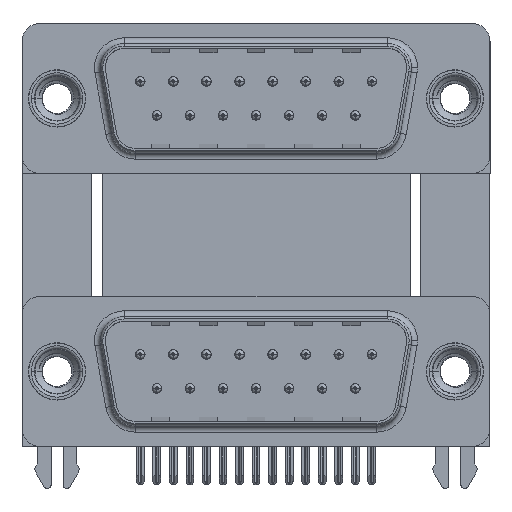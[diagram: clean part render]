
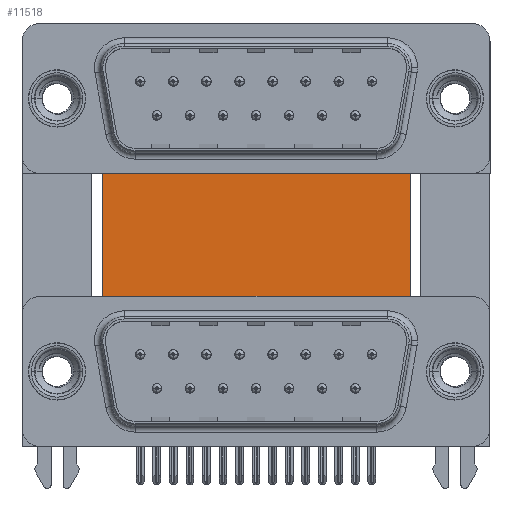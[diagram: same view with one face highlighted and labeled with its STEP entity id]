
A CAD part, top view. The second image highlights one B-rep face of the part: STEP entity #11518.
In plain terms, the highlighted planar face has unit normal (0, 0, 1).
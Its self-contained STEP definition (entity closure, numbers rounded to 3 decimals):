
#62 = VERTEX_POINT ( 'NONE', #31381 ) ;
#1305 = LINE ( 'NONE', #28938, #19242 ) ;
#3365 = CARTESIAN_POINT ( 'NONE',  ( 3.79, 16.585, -12. ) ) ;
#4506 = LINE ( 'NONE', #14262, #23867 ) ;
#5731 = PLANE ( 'NONE',  #9379 ) ;
#6232 = FACE_OUTER_BOUND ( 'NONE', #24358, .T. ) ;
#8092 = DIRECTION ( 'NONE',  ( 0., -1., 0. ) ) ;
#8930 = DIRECTION ( 'NONE',  ( 0., 0., -1. ) ) ;
#9379 = AXIS2_PLACEMENT_3D ( 'NONE', #19197, #8930, #10949 ) ;
#9506 = LINE ( 'NONE', #32763, #24781 ) ;
#10602 = LINE ( 'NONE', #3365, #31676 ) ;
#10753 = EDGE_CURVE ( 'NONE', #26632, #62, #4506, .T. ) ;
#10949 = DIRECTION ( 'NONE',  ( -1., 0., 0. ) ) ;
#11046 = ORIENTED_EDGE ( 'NONE', *, *, #25120, .F. ) ;
#11518 = ADVANCED_FACE ( 'NONE', ( #6232 ), #5731, .F. ) ;
#14262 = CARTESIAN_POINT ( 'NONE',  ( 3.79, -3.735, -12. ) ) ;
#14571 = DIRECTION ( 'NONE',  ( 0., -1., 0. ) ) ;
#14952 = ORIENTED_EDGE ( 'NONE', *, *, #10753, .T. ) ;
#16306 = EDGE_CURVE ( 'NONE', #31346, #26551, #1305, .T. ) ;
#16488 = CARTESIAN_POINT ( 'NONE',  ( 3.79, 16.585, -12. ) ) ;
#16693 = ORIENTED_EDGE ( 'NONE', *, *, #26308, .T. ) ;
#16793 = DIRECTION ( 'NONE',  ( 1., 0., 0. ) ) ;
#17887 = ORIENTED_EDGE ( 'NONE', *, *, #16306, .F. ) ;
#19197 = CARTESIAN_POINT ( 'NONE',  ( 3.79, 16.585, -12. ) ) ;
#19242 = VECTOR ( 'NONE', #16793, 1000. ) ;
#23867 = VECTOR ( 'NONE', #24720, 1000. ) ;
#24358 = EDGE_LOOP ( 'NONE', ( #14952, #11046, #17887, #16693 ) ) ;
#24720 = DIRECTION ( 'NONE',  ( 1., 0., 0. ) ) ;
#24781 = VECTOR ( 'NONE', #14571, 1000. ) ;
#25120 = EDGE_CURVE ( 'NONE', #26551, #62, #9506, .T. ) ;
#26308 = EDGE_CURVE ( 'NONE', #31346, #26632, #10602, .T. ) ;
#26551 = VERTEX_POINT ( 'NONE', #33145 ) ;
#26632 = VERTEX_POINT ( 'NONE', #28602 ) ;
#28602 = CARTESIAN_POINT ( 'NONE',  ( 3.79, -3.735, -12. ) ) ;
#28938 = CARTESIAN_POINT ( 'NONE',  ( 3.79, 16.585, -12. ) ) ;
#31346 = VERTEX_POINT ( 'NONE', #16488 ) ;
#31381 = CARTESIAN_POINT ( 'NONE',  ( 29.58, -3.735, -12. ) ) ;
#31676 = VECTOR ( 'NONE', #8092, 1000. ) ;
#32763 = CARTESIAN_POINT ( 'NONE',  ( 29.58, 16.585, -12. ) ) ;
#33145 = CARTESIAN_POINT ( 'NONE',  ( 29.58, 16.585, -12. ) ) ;
